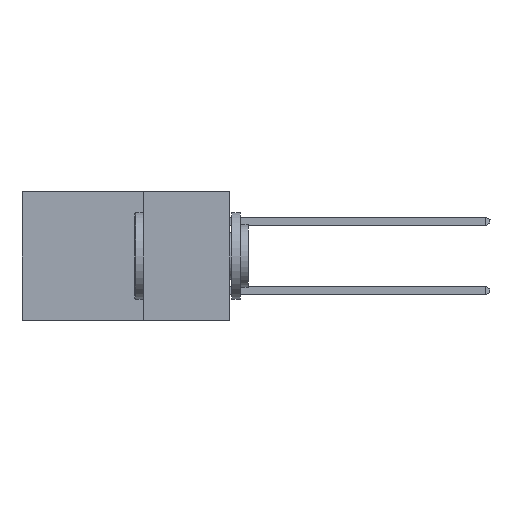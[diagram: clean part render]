
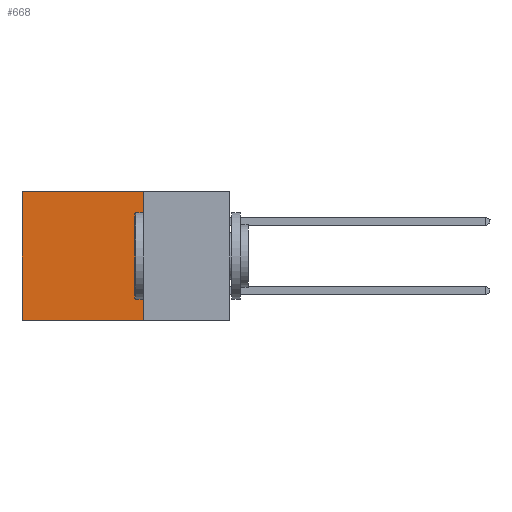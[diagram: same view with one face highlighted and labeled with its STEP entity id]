
A CAD part, left-side view. The second image highlights one B-rep face of the part: STEP entity #668.
In plain terms, the highlighted planar face has unit normal (-1, 0, 0).
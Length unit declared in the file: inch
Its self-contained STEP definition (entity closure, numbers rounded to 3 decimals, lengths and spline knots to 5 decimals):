
#668 = ADVANCED_FACE ( 'NONE', ( #4590 ), #9905, .F. ) ;
#932 = EDGE_CURVE ( 'NONE', #5089, #9129, #2733, .T. ) ;
#975 = DIRECTION ( 'NONE',  ( 0., 1., 0. ) ) ;
#1212 = DIRECTION ( 'NONE',  ( 0., 0., -1. ) ) ;
#1275 = VERTEX_POINT ( 'NONE', #9464 ) ;
#1616 = AXIS2_PLACEMENT_3D ( 'NONE', #7264, #2068, #1212 ) ;
#1705 = ORIENTED_EDGE ( 'NONE', *, *, #10397, .T. ) ;
#1821 = CARTESIAN_POINT ( 'NONE',  ( 0.2615, 0.25, -0.37 ) ) ;
#2068 = DIRECTION ( 'NONE',  ( 1., 0., 0. ) ) ;
#2344 = CARTESIAN_POINT ( 'NONE',  ( 0.2615, 0.25, 0. ) ) ;
#2552 = CARTESIAN_POINT ( 'NONE',  ( 0.2615, 0.25, -0.37 ) ) ;
#2626 = DIRECTION ( 'NONE',  ( 0., 0., -1. ) ) ;
#2667 = LINE ( 'NONE', #2552, #9342 ) ;
#2733 = LINE ( 'NONE', #1821, #8552 ) ;
#3017 = EDGE_LOOP ( 'NONE', ( #1705, #4788, #9015, #8323 ) ) ;
#3919 = VECTOR ( 'NONE', #7392, 39.37008 ) ;
#4590 = FACE_OUTER_BOUND ( 'NONE', #3017, .T. ) ;
#4705 = EDGE_CURVE ( 'NONE', #9129, #1275, #2667, .T. ) ;
#4788 = ORIENTED_EDGE ( 'NONE', *, *, #4705, .F. ) ;
#5085 = LINE ( 'NONE', #8569, #7885 ) ;
#5089 = VERTEX_POINT ( 'NONE', #2344 ) ;
#5410 = CARTESIAN_POINT ( 'NONE',  ( 0.2615, 0.25, -0.37 ) ) ;
#6661 = VERTEX_POINT ( 'NONE', #10717 ) ;
#7243 = EDGE_CURVE ( 'NONE', #5089, #6661, #5085, .T. ) ;
#7264 = CARTESIAN_POINT ( 'NONE',  ( 0.2615, 0.25, -0.37 ) ) ;
#7392 = DIRECTION ( 'NONE',  ( 0., 0., -1. ) ) ;
#7885 = VECTOR ( 'NONE', #975, 39.37008 ) ;
#8323 = ORIENTED_EDGE ( 'NONE', *, *, #7243, .T. ) ;
#8552 = VECTOR ( 'NONE', #2626, 39.37008 ) ;
#8569 = CARTESIAN_POINT ( 'NONE',  ( 0.2615, 0.25, 0. ) ) ;
#8606 = DIRECTION ( 'NONE',  ( 0., 1., 0. ) ) ;
#9015 = ORIENTED_EDGE ( 'NONE', *, *, #932, .F. ) ;
#9129 = VERTEX_POINT ( 'NONE', #5410 ) ;
#9342 = VECTOR ( 'NONE', #8606, 39.37008 ) ;
#9464 = CARTESIAN_POINT ( 'NONE',  ( 0.2615, 0.6, -0.37 ) ) ;
#9905 = PLANE ( 'NONE',  #1616 ) ;
#10397 = EDGE_CURVE ( 'NONE', #6661, #1275, #11042, .T. ) ;
#10717 = CARTESIAN_POINT ( 'NONE',  ( 0.2615, 0.6, 0. ) ) ;
#10817 = CARTESIAN_POINT ( 'NONE',  ( 0.2615, 0.6, -0.37 ) ) ;
#11042 = LINE ( 'NONE', #10817, #3919 ) ;
